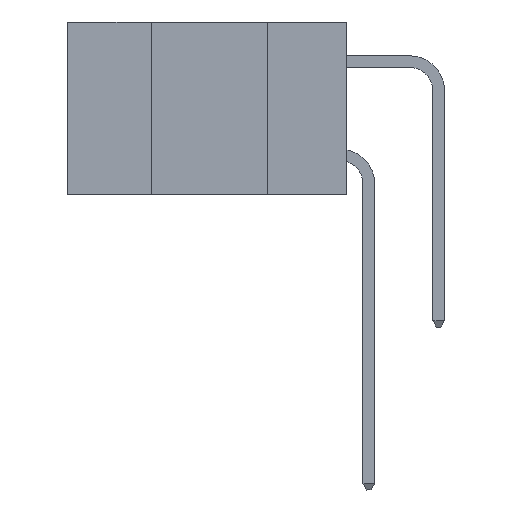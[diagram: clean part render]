
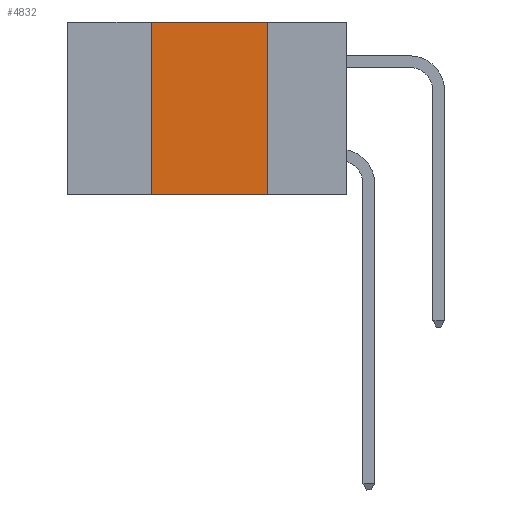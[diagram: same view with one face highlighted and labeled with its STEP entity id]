
A CAD part, left-side view. The second image highlights one B-rep face of the part: STEP entity #4832.
In plain terms, the highlighted planar face has unit normal (-1, 0, 0).
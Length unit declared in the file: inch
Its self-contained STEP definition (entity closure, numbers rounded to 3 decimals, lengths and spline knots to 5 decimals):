
#157 = LINE ( 'NONE', #19791, #9619 ) ;
#1173 = EDGE_CURVE ( 'NONE', #1851, #13573, #6233, .T. ) ;
#1851 = VERTEX_POINT ( 'NONE', #16523 ) ;
#1907 = EDGE_CURVE ( 'NONE', #13257, #1851, #17226, .T. ) ;
#4708 = CARTESIAN_POINT ( 'NONE',  ( 0., 0.6, -0.37 ) ) ;
#4832 = ADVANCED_FACE ( 'NONE', ( #22821 ), #21039, .F. ) ;
#5086 = DIRECTION ( 'NONE',  ( 0., 0., -1. ) ) ;
#6233 = LINE ( 'NONE', #12456, #20475 ) ;
#6586 = DIRECTION ( 'NONE',  ( 0., -1., 0. ) ) ;
#7374 = VECTOR ( 'NONE', #9362, 39.37008 ) ;
#7462 = CARTESIAN_POINT ( 'NONE',  ( 0., 0.6, 0. ) ) ;
#8050 = VERTEX_POINT ( 'NONE', #12417 ) ;
#9362 = DIRECTION ( 'NONE',  ( 0., -1., 0. ) ) ;
#9375 = ORIENTED_EDGE ( 'NONE', *, *, #1907, .F. ) ;
#9619 = VECTOR ( 'NONE', #21654, 39.37008 ) ;
#10106 = EDGE_LOOP ( 'NONE', ( #10221, #9375, #13368, #11927 ) ) ;
#10221 = ORIENTED_EDGE ( 'NONE', *, *, #1173, .F. ) ;
#11729 = DIRECTION ( 'NONE',  ( 0., 0., -1. ) ) ;
#11927 = ORIENTED_EDGE ( 'NONE', *, *, #17585, .T. ) ;
#12166 = CARTESIAN_POINT ( 'NONE',  ( 0., 0.42, 0. ) ) ;
#12417 = CARTESIAN_POINT ( 'NONE',  ( 0., 0.42, -0.37 ) ) ;
#12456 = CARTESIAN_POINT ( 'NONE',  ( 0., 0.17, 0. ) ) ;
#13257 = VERTEX_POINT ( 'NONE', #12166 ) ;
#13368 = ORIENTED_EDGE ( 'NONE', *, *, #21648, .F. ) ;
#13573 = VERTEX_POINT ( 'NONE', #24137 ) ;
#13817 = LINE ( 'NONE', #4708, #23119 ) ;
#16523 = CARTESIAN_POINT ( 'NONE',  ( 0., 0.17, 0. ) ) ;
#17226 = LINE ( 'NONE', #7462, #7374 ) ;
#17267 = CARTESIAN_POINT ( 'NONE',  ( 0., 0.6, 0. ) ) ;
#17585 = EDGE_CURVE ( 'NONE', #8050, #13573, #13817, .T. ) ;
#19791 = CARTESIAN_POINT ( 'NONE',  ( 0., 0.42, 0. ) ) ;
#20475 = VECTOR ( 'NONE', #5086, 39.37008 ) ;
#20747 = AXIS2_PLACEMENT_3D ( 'NONE', #17267, #22872, #11729 ) ;
#21039 = PLANE ( 'NONE',  #20747 ) ;
#21648 = EDGE_CURVE ( 'NONE', #8050, #13257, #157, .T. ) ;
#21654 = DIRECTION ( 'NONE',  ( 0., 0., 1. ) ) ;
#22821 = FACE_OUTER_BOUND ( 'NONE', #10106, .T. ) ;
#22872 = DIRECTION ( 'NONE',  ( 1., 0., 0. ) ) ;
#23119 = VECTOR ( 'NONE', #6586, 39.37008 ) ;
#24137 = CARTESIAN_POINT ( 'NONE',  ( 0., 0.17, -0.37 ) ) ;
